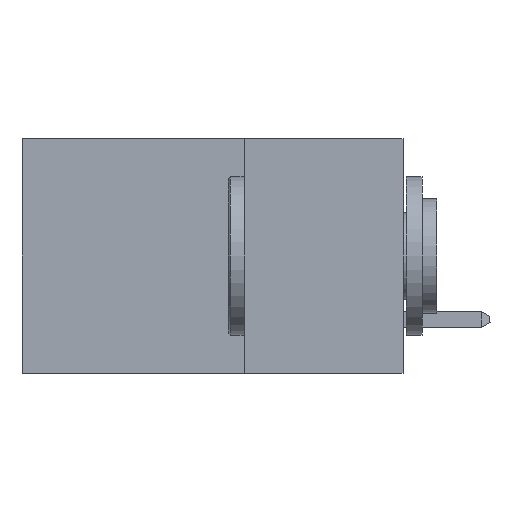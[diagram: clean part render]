
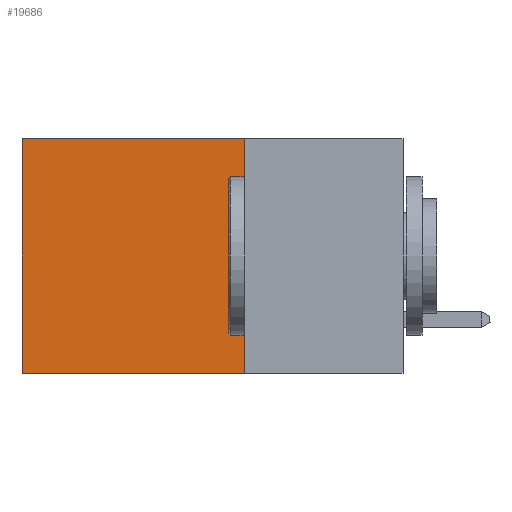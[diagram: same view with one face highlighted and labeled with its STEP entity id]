
A CAD part, left-side view. The second image highlights one B-rep face of the part: STEP entity #19686.
In plain terms, the highlighted planar face has unit normal (-1, 0, 0).
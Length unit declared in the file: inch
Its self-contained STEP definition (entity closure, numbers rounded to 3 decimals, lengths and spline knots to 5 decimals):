
#2702 = DIRECTION ( 'NONE',  ( 0., 1., 0. ) ) ;
#5071 = AXIS2_PLACEMENT_3D ( 'NONE', #11904, #12515, #29344 ) ;
#5391 = ORIENTED_EDGE ( 'NONE', *, *, #29423, .F. ) ;
#7571 = VERTEX_POINT ( 'NONE', #11336 ) ;
#8498 = PLANE ( 'NONE',  #5071 ) ;
#8605 = EDGE_CURVE ( 'NONE', #7571, #39399, #35504, .T. ) ;
#9664 = VERTEX_POINT ( 'NONE', #11279 ) ;
#9905 = EDGE_CURVE ( 'NONE', #26554, #7571, #23751, .T. ) ;
#10925 = FACE_OUTER_BOUND ( 'NONE', #30969, .T. ) ;
#11279 = CARTESIAN_POINT ( 'NONE',  ( 0.2875, 0.25, -0.37 ) ) ;
#11336 = CARTESIAN_POINT ( 'NONE',  ( 0.2875, 0.6, 0. ) ) ;
#11904 = CARTESIAN_POINT ( 'NONE',  ( 0.2875, 0.25, 0. ) ) ;
#12515 = DIRECTION ( 'NONE',  ( 1., 0., 0. ) ) ;
#13685 = ORIENTED_EDGE ( 'NONE', *, *, #9905, .T. ) ;
#14285 = CARTESIAN_POINT ( 'NONE',  ( 0.2875, 0.6, 0. ) ) ;
#14601 = CARTESIAN_POINT ( 'NONE',  ( 0.2875, 0.25, 0. ) ) ;
#16456 = VECTOR ( 'NONE', #21236, 39.37008 ) ;
#19260 = VECTOR ( 'NONE', #2702, 39.37008 ) ;
#19686 = ADVANCED_FACE ( 'NONE', ( #10925 ), #8498, .F. ) ;
#20260 = LINE ( 'NONE', #41713, #19260 ) ;
#20784 = CARTESIAN_POINT ( 'NONE',  ( 0.2875, 0.25, 0. ) ) ;
#21236 = DIRECTION ( 'NONE',  ( 0., 1., 0. ) ) ;
#23731 = VECTOR ( 'NONE', #25014, 39.37008 ) ;
#23751 = LINE ( 'NONE', #20784, #16456 ) ;
#24403 = DIRECTION ( 'NONE',  ( 0., 0., -1. ) ) ;
#24757 = ORIENTED_EDGE ( 'NONE', *, *, #8605, .T. ) ;
#25014 = DIRECTION ( 'NONE',  ( 0., 0., -1. ) ) ;
#25955 = EDGE_CURVE ( 'NONE', #9664, #39399, #20260, .T. ) ;
#26177 = CARTESIAN_POINT ( 'NONE',  ( 0.2875, 0.6, -0.37 ) ) ;
#26554 = VERTEX_POINT ( 'NONE', #34271 ) ;
#29344 = DIRECTION ( 'NONE',  ( 0., 0., -1. ) ) ;
#29423 = EDGE_CURVE ( 'NONE', #26554, #9664, #35741, .T. ) ;
#29476 = ORIENTED_EDGE ( 'NONE', *, *, #25955, .F. ) ;
#30969 = EDGE_LOOP ( 'NONE', ( #24757, #29476, #5391, #13685 ) ) ;
#34271 = CARTESIAN_POINT ( 'NONE',  ( 0.2875, 0.25, 0. ) ) ;
#35504 = LINE ( 'NONE', #14285, #39700 ) ;
#35741 = LINE ( 'NONE', #14601, #23731 ) ;
#39399 = VERTEX_POINT ( 'NONE', #26177 ) ;
#39700 = VECTOR ( 'NONE', #24403, 39.37008 ) ;
#41713 = CARTESIAN_POINT ( 'NONE',  ( 0.2875, 0.25, -0.37 ) ) ;
